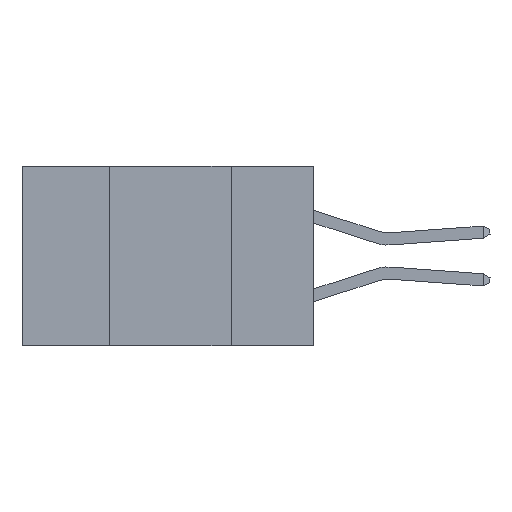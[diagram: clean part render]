
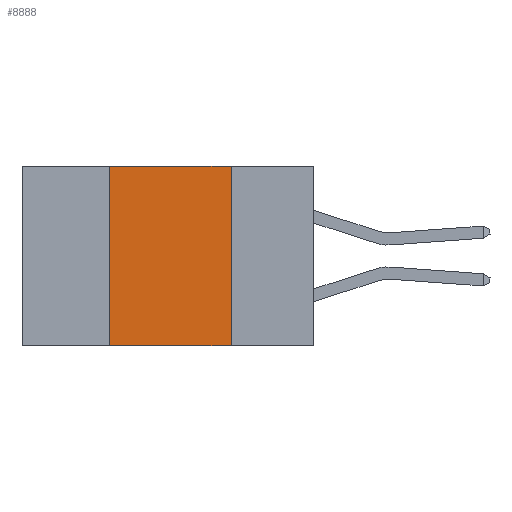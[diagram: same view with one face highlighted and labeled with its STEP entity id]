
A CAD part, left-side view. The second image highlights one B-rep face of the part: STEP entity #8888.
In plain terms, the highlighted planar face has unit normal (-1, 0, 0).
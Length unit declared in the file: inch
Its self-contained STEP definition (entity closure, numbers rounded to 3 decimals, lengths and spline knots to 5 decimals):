
#619 = LINE ( 'NONE', #8246, #6432 ) ;
#1242 = VECTOR ( 'NONE', #8534, 39.37008 ) ;
#1454 = CARTESIAN_POINT ( 'NONE',  ( 0., 0.42, -0.37 ) ) ;
#1494 = LINE ( 'NONE', #5186, #3231 ) ;
#1712 = ORIENTED_EDGE ( 'NONE', *, *, #9270, .T. ) ;
#2322 = FACE_OUTER_BOUND ( 'NONE', #7056, .T. ) ;
#2556 = LINE ( 'NONE', #3253, #6392 ) ;
#3092 = DIRECTION ( 'NONE',  ( 1., 0., 0. ) ) ;
#3212 = ORIENTED_EDGE ( 'NONE', *, *, #5042, .F. ) ;
#3231 = VECTOR ( 'NONE', #5957, 39.37008 ) ;
#3253 = CARTESIAN_POINT ( 'NONE',  ( 0., 0.42, 0. ) ) ;
#3430 = LINE ( 'NONE', #8572, #1242 ) ;
#3640 = VERTEX_POINT ( 'NONE', #8617 ) ;
#3737 = AXIS2_PLACEMENT_3D ( 'NONE', #6169, #3092, #8429 ) ;
#3932 = EDGE_CURVE ( 'NONE', #4114, #3640, #3430, .T. ) ;
#3997 = DIRECTION ( 'NONE',  ( 0., 0., 1. ) ) ;
#4114 = VERTEX_POINT ( 'NONE', #5969 ) ;
#4599 = VERTEX_POINT ( 'NONE', #6041 ) ;
#5042 = EDGE_CURVE ( 'NONE', #4599, #4114, #619, .T. ) ;
#5186 = CARTESIAN_POINT ( 'NONE',  ( 0., 0.6, -0.37 ) ) ;
#5957 = DIRECTION ( 'NONE',  ( 0., -1., 0. ) ) ;
#5969 = CARTESIAN_POINT ( 'NONE',  ( 0., 0.17, 0. ) ) ;
#6041 = CARTESIAN_POINT ( 'NONE',  ( 0., 0.42, 0. ) ) ;
#6169 = CARTESIAN_POINT ( 'NONE',  ( 0., 0.6, 0. ) ) ;
#6392 = VECTOR ( 'NONE', #3997, 39.37008 ) ;
#6432 = VECTOR ( 'NONE', #6932, 39.37008 ) ;
#6460 = EDGE_CURVE ( 'NONE', #8098, #4599, #2556, .T. ) ;
#6901 = PLANE ( 'NONE',  #3737 ) ;
#6932 = DIRECTION ( 'NONE',  ( 0., -1., 0. ) ) ;
#7013 = ORIENTED_EDGE ( 'NONE', *, *, #3932, .F. ) ;
#7056 = EDGE_LOOP ( 'NONE', ( #7013, #3212, #9475, #1712 ) ) ;
#8098 = VERTEX_POINT ( 'NONE', #1454 ) ;
#8246 = CARTESIAN_POINT ( 'NONE',  ( 0., 0.6, 0. ) ) ;
#8429 = DIRECTION ( 'NONE',  ( 0., 0., -1. ) ) ;
#8534 = DIRECTION ( 'NONE',  ( 0., 0., -1. ) ) ;
#8572 = CARTESIAN_POINT ( 'NONE',  ( 0., 0.17, 0. ) ) ;
#8617 = CARTESIAN_POINT ( 'NONE',  ( 0., 0.17, -0.37 ) ) ;
#8888 = ADVANCED_FACE ( 'NONE', ( #2322 ), #6901, .F. ) ;
#9270 = EDGE_CURVE ( 'NONE', #8098, #3640, #1494, .T. ) ;
#9475 = ORIENTED_EDGE ( 'NONE', *, *, #6460, .F. ) ;
